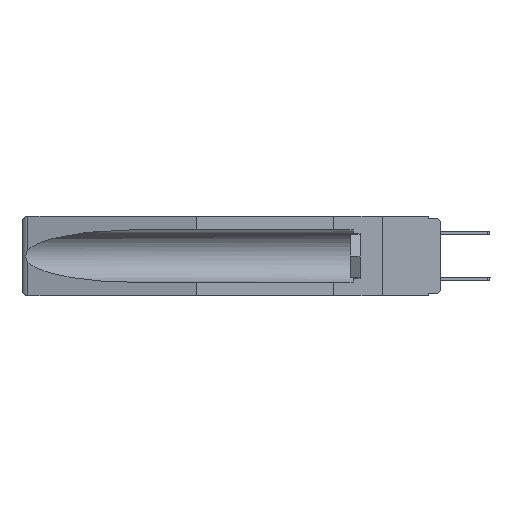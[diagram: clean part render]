
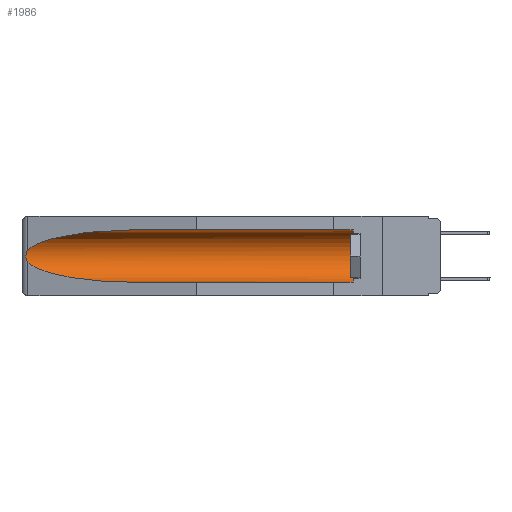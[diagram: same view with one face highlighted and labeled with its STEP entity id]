
A CAD part, left-side view. The second image highlights one B-rep face of the part: STEP entity #1986.
In plain terms, the highlighted cylindrical face has radius 2.857 mm (diameter 5.715 mm), a partial arc.
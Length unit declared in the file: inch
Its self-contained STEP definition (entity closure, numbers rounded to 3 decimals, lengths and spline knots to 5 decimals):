
#642 = CARTESIAN_POINT ( 'NONE',  ( 0.26537, 1.52718, -0.14972 ) ) ;
#822 = CARTESIAN_POINT ( 'NONE',  ( 0.26537, 1.52718, -0.14972 ) ) ;
#973 = CARTESIAN_POINT ( 'NONE',  ( 0.25451, 1.48313, -0.09465 ) ) ;
#1103 = CARTESIAN_POINT ( 'NONE',  ( 0.26597, 1.5296, -0.19026 ) ) ;
#1986 = ADVANCED_FACE ( 'NONE', ( #13670 ), #8973, .F. ) ;
#2043 = CARTESIAN_POINT ( 'NONE',  ( 0.155, 0.126, -0.059 ) ) ;
#2179 = CARTESIAN_POINT ( 'NONE',  ( 0.155, 1.07973, -0.059 ) ) ;
#2793 = CARTESIAN_POINT ( 'NONE',  ( 0.155, 1.07973, -0.284 ) ) ;
#3270 = DIRECTION ( 'NONE',  ( 0., 1., 0. ) ) ;
#3476 = EDGE_CURVE ( 'NONE', #19351, #3536, #22711, .T. ) ;
#3536 = VERTEX_POINT ( 'NONE', #5174 ) ;
#3567 = ORIENTED_EDGE ( 'NONE', *, *, #8259, .T. ) ;
#3647 = CIRCLE ( 'NONE', #17689, 0.1125 ) ;
#3837 = VECTOR ( 'NONE', #20383, 39.37008 ) ;
#3858 = LINE ( 'NONE', #4357, #3837 ) ;
#4311 = CARTESIAN_POINT ( 'NONE',  ( 0.21114, 1.30732, -0.059 ) ) ;
#4357 = CARTESIAN_POINT ( 'NONE',  ( 0.155, -0.30754, -0.059 ) ) ;
#4442 = CARTESIAN_POINT ( 'NONE',  ( 0.2675, 1.53308, -0.16763 ) ) ;
#4513 = CARTESIAN_POINT ( 'NONE',  ( 0.26655, 1.53094, -0.18657 ) ) ;
#4951 = CARTESIAN_POINT ( 'NONE',  ( 0.155, -0.30754, -0.284 ) ) ;
#5174 = CARTESIAN_POINT ( 'NONE',  ( 0.155, 1.07973, -0.284 ) ) ;
#6107 = DIRECTION ( 'NONE',  ( 0., 0., 1. ) ) ;
#6245 = CARTESIAN_POINT ( 'NONE',  ( 0.26537, 1.52718, -0.19328 ) ) ;
#6250 = VERTEX_POINT ( 'NONE', #2179 ) ;
#7911 = CARTESIAN_POINT ( 'NONE',  ( 0.2673, 1.5327, -0.16383 ) ) ;
#8259 = EDGE_CURVE ( 'NONE', #19351, #21837, #3647, .T. ) ;
#8325 = EDGE_CURVE ( 'NONE', #21837, #6250, #3858, .T. ) ;
#8973 = CYLINDRICAL_SURFACE ( 'NONE', #19400, 0.1125 ) ;
#9408 = VERTEX_POINT ( 'NONE', #20561 ) ;
#9485 = CARTESIAN_POINT ( 'NONE',  ( 0.26537, 1.52718, -0.14972 ) ) ;
#10041 = CARTESIAN_POINT ( 'NONE',  ( 0.26654, 1.53092, -0.15636 ) ) ;
#10327 =( BOUNDED_CURVE ( )  B_SPLINE_CURVE ( 3, ( #6245, #22210, #20439, #2793 ),
 .UNSPECIFIED., .F., .F. ) 
 B_SPLINE_CURVE_WITH_KNOTS ( ( 4, 4 ),
 ( 0.1948, 1.5708 ),
 .UNSPECIFIED. ) 
 CURVE ( )  GEOMETRIC_REPRESENTATION_ITEM ( )  RATIONAL_B_SPLINE_CURVE ( ( 1., 0.848, 0.848, 1. ) ) 
 REPRESENTATION_ITEM ( '' )  );
#10735 = ORIENTED_EDGE ( 'NONE', *, *, #8325, .T. ) ;
#10797 = DIRECTION ( 'NONE',  ( 0., 0., 1. ) ) ;
#10971 = EDGE_CURVE ( 'NONE', #9408, #3536, #10327, .T. ) ;
#11643 = ORIENTED_EDGE ( 'NONE', *, *, #20837, .T. ) ;
#11918 = VECTOR ( 'NONE', #3270, 39.37008 ) ;
#13431 = B_SPLINE_CURVE_WITH_KNOTS ( 'NONE', 3,
 ( #9485, #21862, #10041, #7911, #4442, #15101, #18591, #4513, #1103, #17036 ),
 .UNSPECIFIED., .F., .F.,
 ( 4, 2, 2, 2, 4 ),
 ( 0., 0.00029, 0.00058, 0.00087, 0.00117 ),
 .UNSPECIFIED. ) ;
#13512 = VERTEX_POINT ( 'NONE', #642 ) ;
#13670 = FACE_OUTER_BOUND ( 'NONE', #18245, .T. ) ;
#14553 = CARTESIAN_POINT ( 'NONE',  ( 0.155, 0.126, -0.284 ) ) ;
#14777 = ORIENTED_EDGE ( 'NONE', *, *, #20197, .T. ) ;
#14824 = CARTESIAN_POINT ( 'NONE',  ( 0.155, 1.07973, -0.059 ) ) ;
#15101 = CARTESIAN_POINT ( 'NONE',  ( 0.2675, 1.53308, -0.17534 ) ) ;
#15785 = ORIENTED_EDGE ( 'NONE', *, *, #3476, .F. ) ;
#16876 = DIRECTION ( 'NONE',  ( 0., -1., 0. ) ) ;
#17036 = CARTESIAN_POINT ( 'NONE',  ( 0.26537, 1.52718, -0.19328 ) ) ;
#17510 =( BOUNDED_CURVE ( )  B_SPLINE_CURVE ( 3, ( #14824, #4311, #973, #822 ),
 .UNSPECIFIED., .F., .F. ) 
 B_SPLINE_CURVE_WITH_KNOTS ( ( 4, 4 ),
 ( 4.71239, 6.08839 ),
 .UNSPECIFIED. ) 
 CURVE ( )  GEOMETRIC_REPRESENTATION_ITEM ( )  RATIONAL_B_SPLINE_CURVE ( ( 1., 0.848, 0.848, 1. ) ) 
 REPRESENTATION_ITEM ( '' )  );
#17689 = AXIS2_PLACEMENT_3D ( 'NONE', #18661, #16876, #6107 ) ;
#18245 = EDGE_LOOP ( 'NONE', ( #14777, #11643, #20883, #15785, #3567, #10735 ) ) ;
#18591 = CARTESIAN_POINT ( 'NONE',  ( 0.2673, 1.53269, -0.17917 ) ) ;
#18661 = CARTESIAN_POINT ( 'NONE',  ( 0.155, 0.126, -0.1715 ) ) ;
#19351 = VERTEX_POINT ( 'NONE', #14553 ) ;
#19400 = AXIS2_PLACEMENT_3D ( 'NONE', #21553, #19605, #10797 ) ;
#19605 = DIRECTION ( 'NONE',  ( 0., 1., 0. ) ) ;
#20197 = EDGE_CURVE ( 'NONE', #6250, #13512, #17510, .T. ) ;
#20383 = DIRECTION ( 'NONE',  ( 0., 1., 0. ) ) ;
#20439 = CARTESIAN_POINT ( 'NONE',  ( 0.21114, 1.30732, -0.284 ) ) ;
#20561 = CARTESIAN_POINT ( 'NONE',  ( 0.26537, 1.52718, -0.19328 ) ) ;
#20837 = EDGE_CURVE ( 'NONE', #13512, #9408, #13431, .T. ) ;
#20883 = ORIENTED_EDGE ( 'NONE', *, *, #10971, .T. ) ;
#21553 = CARTESIAN_POINT ( 'NONE',  ( 0.155, -0.30754, -0.1715 ) ) ;
#21837 = VERTEX_POINT ( 'NONE', #2043 ) ;
#21862 = CARTESIAN_POINT ( 'NONE',  ( 0.26597, 1.52961, -0.15275 ) ) ;
#22210 = CARTESIAN_POINT ( 'NONE',  ( 0.25451, 1.48313, -0.24835 ) ) ;
#22711 = LINE ( 'NONE', #4951, #11918 ) ;
